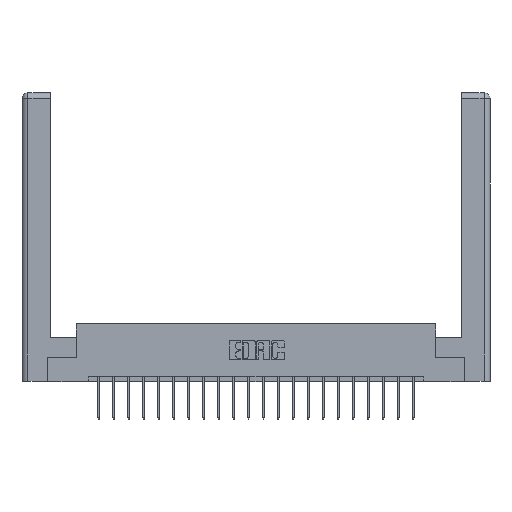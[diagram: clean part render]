
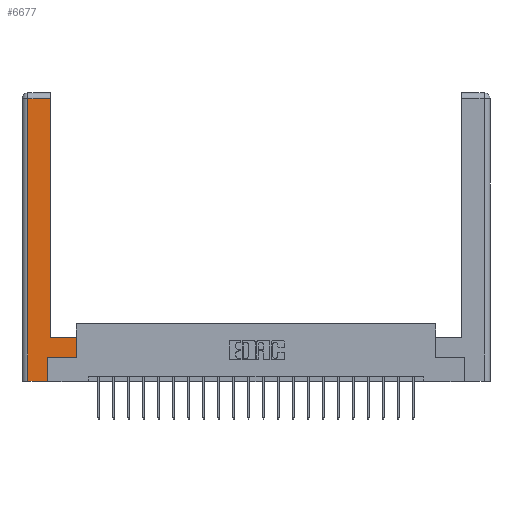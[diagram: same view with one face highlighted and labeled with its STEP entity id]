
A CAD part, top view. The second image highlights one B-rep face of the part: STEP entity #6677.
In plain terms, the highlighted planar face has unit normal (0, 0, 1).
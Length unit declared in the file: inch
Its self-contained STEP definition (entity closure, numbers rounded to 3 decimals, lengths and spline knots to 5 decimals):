
#113 = ORIENTED_EDGE ( 'NONE', *, *, #8010, .T. ) ;
#366 = CARTESIAN_POINT ( 'NONE',  ( 0.295, 3., 0. ) ) ;
#414 = CARTESIAN_POINT ( 'NONE',  ( 0.565, 0.245, 0. ) ) ;
#1401 = PLANE ( 'NONE',  #15665 ) ;
#1481 = EDGE_CURVE ( 'NONE', #19985, #15250, #22098, .T. ) ;
#1538 = VERTEX_POINT ( 'NONE', #18330 ) ;
#1593 = FACE_OUTER_BOUND ( 'NONE', #16576, .T. ) ;
#1628 = LINE ( 'NONE', #3971, #19475 ) ;
#1836 = CARTESIAN_POINT ( 'NONE',  ( 0.0615, 0., 0. ) ) ;
#2300 = DIRECTION ( 'NONE',  ( 0., 1., 0. ) ) ;
#2716 = DIRECTION ( 'NONE',  ( -1., 0., 0. ) ) ;
#3101 = CARTESIAN_POINT ( 'NONE',  ( 0.295, 2.94, 0. ) ) ;
#3197 = VECTOR ( 'NONE', #11346, 39.37008 ) ;
#3199 = CARTESIAN_POINT ( 'NONE',  ( 0.295, 0.45, 0. ) ) ;
#3409 = ORIENTED_EDGE ( 'NONE', *, *, #7061, .T. ) ;
#3619 = VERTEX_POINT ( 'NONE', #1836 ) ;
#3971 = CARTESIAN_POINT ( 'NONE',  ( 0.265, 0.245, 0. ) ) ;
#4048 = EDGE_CURVE ( 'NONE', #12818, #19985, #16290, .T. ) ;
#4251 = EDGE_CURVE ( 'NONE', #15250, #11868, #14918, .T. ) ;
#4252 = LINE ( 'NONE', #7081, #22089 ) ;
#4537 = ORIENTED_EDGE ( 'NONE', *, *, #13042, .T. ) ;
#4921 = VECTOR ( 'NONE', #2300, 39.37008 ) ;
#5205 = EDGE_CURVE ( 'NONE', #16287, #8156, #1628, .T. ) ;
#6360 = DIRECTION ( 'NONE',  ( 0., 1., 0. ) ) ;
#6420 = VECTOR ( 'NONE', #2716, 39.37008 ) ;
#6677 = ADVANCED_FACE ( 'NONE', ( #1593 ), #1401, .F. ) ;
#7061 = EDGE_CURVE ( 'NONE', #8156, #12818, #12401, .T. ) ;
#7081 = CARTESIAN_POINT ( 'NONE',  ( 0.265, 0., 0. ) ) ;
#8010 = EDGE_CURVE ( 'NONE', #3619, #16287, #4252, .T. ) ;
#8156 = VERTEX_POINT ( 'NONE', #19851 ) ;
#8221 = ORIENTED_EDGE ( 'NONE', *, *, #5205, .T. ) ;
#8933 = ORIENTED_EDGE ( 'NONE', *, *, #11989, .T. ) ;
#9134 = DIRECTION ( 'NONE',  ( 0., 1., 0. ) ) ;
#9421 = DIRECTION ( 'NONE',  ( -1., 0., 0. ) ) ;
#9578 = CARTESIAN_POINT ( 'NONE',  ( 0.295, 0.45, 0. ) ) ;
#9609 = CARTESIAN_POINT ( 'NONE',  ( 0.565, 0.245, 0. ) ) ;
#10080 = CARTESIAN_POINT ( 'NONE',  ( 0., 0., 0. ) ) ;
#10602 = VECTOR ( 'NONE', #6360, 39.37008 ) ;
#10681 = DIRECTION ( 'NONE',  ( 0., -1., 0. ) ) ;
#11346 = DIRECTION ( 'NONE',  ( 1., 0., 0. ) ) ;
#11709 = ORIENTED_EDGE ( 'NONE', *, *, #4251, .T. ) ;
#11806 = DIRECTION ( 'NONE',  ( 0., 0., -1. ) ) ;
#11868 = VERTEX_POINT ( 'NONE', #3101 ) ;
#11989 = EDGE_CURVE ( 'NONE', #1538, #3619, #14873, .T. ) ;
#12401 = LINE ( 'NONE', #9609, #3197 ) ;
#12679 = CARTESIAN_POINT ( 'NONE',  ( 0.265, 0., 0. ) ) ;
#12818 = VERTEX_POINT ( 'NONE', #414 ) ;
#13042 = EDGE_CURVE ( 'NONE', #11868, #1538, #20011, .T. ) ;
#14268 = VECTOR ( 'NONE', #9421, 39.37008 ) ;
#14873 = LINE ( 'NONE', #15641, #21690 ) ;
#14918 = LINE ( 'NONE', #366, #4921 ) ;
#15250 = VERTEX_POINT ( 'NONE', #3199 ) ;
#15641 = CARTESIAN_POINT ( 'NONE',  ( 0.0615, 0., 0. ) ) ;
#15665 = AXIS2_PLACEMENT_3D ( 'NONE', #10080, #11806, #17377 ) ;
#15963 = DIRECTION ( 'NONE',  ( 1., 0., 0. ) ) ;
#16287 = VERTEX_POINT ( 'NONE', #12679 ) ;
#16290 = LINE ( 'NONE', #18429, #10602 ) ;
#16576 = EDGE_LOOP ( 'NONE', ( #11709, #4537, #8933, #113, #8221, #3409, #22059, #21315 ) ) ;
#17377 = DIRECTION ( 'NONE',  ( -1., 0., 0. ) ) ;
#18330 = CARTESIAN_POINT ( 'NONE',  ( 0.0615, 2.94, 0. ) ) ;
#18429 = CARTESIAN_POINT ( 'NONE',  ( 0.565, 0.45, 0. ) ) ;
#19475 = VECTOR ( 'NONE', #9134, 39.37008 ) ;
#19851 = CARTESIAN_POINT ( 'NONE',  ( 0.265, 0.245, 0. ) ) ;
#19947 = CARTESIAN_POINT ( 'NONE',  ( 0.0615, 2.94, 0. ) ) ;
#19985 = VERTEX_POINT ( 'NONE', #22244 ) ;
#20011 = LINE ( 'NONE', #19947, #14268 ) ;
#21315 = ORIENTED_EDGE ( 'NONE', *, *, #1481, .T. ) ;
#21690 = VECTOR ( 'NONE', #10681, 39.37008 ) ;
#22059 = ORIENTED_EDGE ( 'NONE', *, *, #4048, .T. ) ;
#22089 = VECTOR ( 'NONE', #15963, 39.37008 ) ;
#22098 = LINE ( 'NONE', #9578, #6420 ) ;
#22244 = CARTESIAN_POINT ( 'NONE',  ( 0.565, 0.45, 0. ) ) ;
